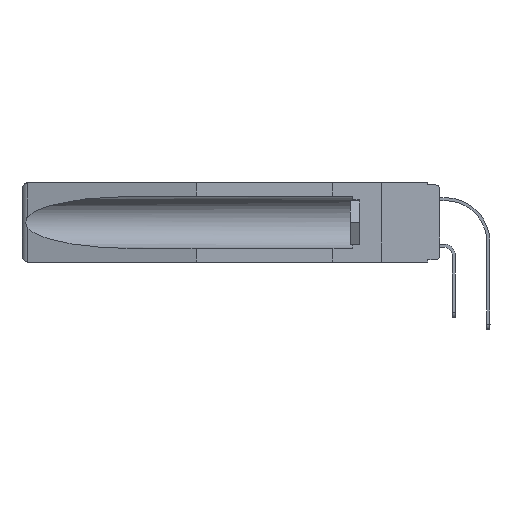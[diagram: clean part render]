
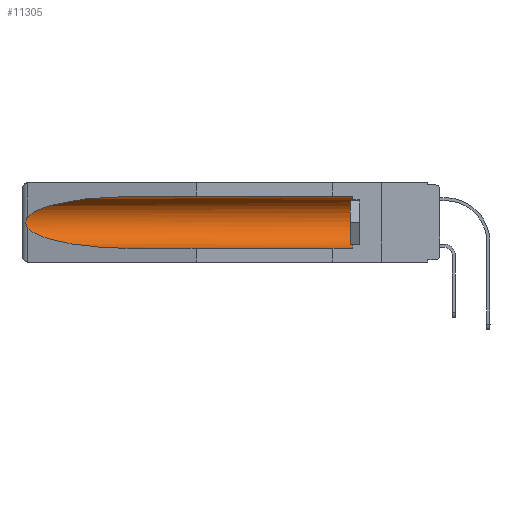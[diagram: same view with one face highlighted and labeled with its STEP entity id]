
A CAD part, left-side view. The second image highlights one B-rep face of the part: STEP entity #11305.
In plain terms, the highlighted cylindrical face has radius 2.857 mm (diameter 5.715 mm), a partial arc.
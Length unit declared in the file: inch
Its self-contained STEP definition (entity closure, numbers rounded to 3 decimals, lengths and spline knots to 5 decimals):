
#684 = CARTESIAN_POINT ( 'NONE',  ( 0.26597, 1.52961, -0.15275 ) ) ;
#916 = CARTESIAN_POINT ( 'NONE',  ( 0.26537, 1.52718, -0.19328 ) ) ;
#1855 = EDGE_CURVE ( 'NONE', #12677, #8878, #17461, .T. ) ;
#2428 = VECTOR ( 'NONE', #4899, 39.37008 ) ;
#2556 = VECTOR ( 'NONE', #22938, 39.37008 ) ;
#2964 = DIRECTION ( 'NONE',  ( 0., -1., 0. ) ) ;
#3357 = CARTESIAN_POINT ( 'NONE',  ( 0.26537, 1.52718, -0.14972 ) ) ;
#3511 = VERTEX_POINT ( 'NONE', #21932 ) ;
#4125 = CIRCLE ( 'NONE', #6401, 0.1125 ) ;
#4135 = EDGE_CURVE ( 'NONE', #6218, #3511, #13485, .T. ) ;
#4216 = CARTESIAN_POINT ( 'NONE',  ( 0.21114, 1.30732, -0.059 ) ) ;
#4338 = CARTESIAN_POINT ( 'NONE',  ( 0.25451, 1.48313, -0.09465 ) ) ;
#4899 = DIRECTION ( 'NONE',  ( 0., 1., 0. ) ) ;
#6130 = EDGE_CURVE ( 'NONE', #12677, #6218, #4125, .T. ) ;
#6218 = VERTEX_POINT ( 'NONE', #7567 ) ;
#6301 = CARTESIAN_POINT ( 'NONE',  ( 0.2673, 1.5327, -0.16383 ) ) ;
#6401 = AXIS2_PLACEMENT_3D ( 'NONE', #8334, #2964, #23059 ) ;
#6752 = CARTESIAN_POINT ( 'NONE',  ( 0.155, 0.126, -0.284 ) ) ;
#7068 = CARTESIAN_POINT ( 'NONE',  ( 0.21114, 1.30732, -0.284 ) ) ;
#7211 = ORIENTED_EDGE ( 'NONE', *, *, #4135, .T. ) ;
#7567 = CARTESIAN_POINT ( 'NONE',  ( 0.155, 0.126, -0.059 ) ) ;
#7980 = CARTESIAN_POINT ( 'NONE',  ( 0.26654, 1.53092, -0.15636 ) ) ;
#8334 = CARTESIAN_POINT ( 'NONE',  ( 0.155, 0.126, -0.1715 ) ) ;
#8448 = CARTESIAN_POINT ( 'NONE',  ( 0.155, -0.30754, -0.059 ) ) ;
#8683 = ORIENTED_EDGE ( 'NONE', *, *, #1855, .F. ) ;
#8878 = VERTEX_POINT ( 'NONE', #14005 ) ;
#8950 = VERTEX_POINT ( 'NONE', #3357 ) ;
#10060 = ORIENTED_EDGE ( 'NONE', *, *, #20190, .T. ) ;
#10434 = ORIENTED_EDGE ( 'NONE', *, *, #13040, .T. ) ;
#10481 = EDGE_LOOP ( 'NONE', ( #10434, #10060, #18855, #8683, #18354, #7211 ) ) ;
#11305 = ADVANCED_FACE ( 'NONE', ( #13354 ), #11776, .F. ) ;
#11628 = CARTESIAN_POINT ( 'NONE',  ( 0.26537, 1.52718, -0.14972 ) ) ;
#11776 = CYLINDRICAL_SURFACE ( 'NONE', #15337, 0.1125 ) ;
#11869 = CARTESIAN_POINT ( 'NONE',  ( 0.155, 1.07973, -0.059 ) ) ;
#12677 = VERTEX_POINT ( 'NONE', #6752 ) ;
#12902 = CARTESIAN_POINT ( 'NONE',  ( 0.26537, 1.52718, -0.19328 ) ) ;
#13040 = EDGE_CURVE ( 'NONE', #3511, #8950, #21766, .T. ) ;
#13354 = FACE_OUTER_BOUND ( 'NONE', #10481, .T. ) ;
#13461 = CARTESIAN_POINT ( 'NONE',  ( 0.155, -0.30754, -0.1715 ) ) ;
#13485 = LINE ( 'NONE', #8448, #2556 ) ;
#13492 = CARTESIAN_POINT ( 'NONE',  ( 0.26655, 1.53094, -0.18657 ) ) ;
#14005 = CARTESIAN_POINT ( 'NONE',  ( 0.155, 1.07973, -0.284 ) ) ;
#14249 = CARTESIAN_POINT ( 'NONE',  ( 0.155, 1.07973, -0.284 ) ) ;
#15279 = CARTESIAN_POINT ( 'NONE',  ( 0.2675, 1.53308, -0.16763 ) ) ;
#15337 = AXIS2_PLACEMENT_3D ( 'NONE', #13461, #15366, #20761 ) ;
#15366 = DIRECTION ( 'NONE',  ( 0., 1., 0. ) ) ;
#15400 = CARTESIAN_POINT ( 'NONE',  ( 0.26537, 1.52718, -0.14972 ) ) ;
#15928 = CARTESIAN_POINT ( 'NONE',  ( 0.26537, 1.52718, -0.19328 ) ) ;
#16098 =( BOUNDED_CURVE ( )  B_SPLINE_CURVE ( 3, ( #15928, #17968, #7068, #14249 ),
 .UNSPECIFIED., .F., .T. ) 
 B_SPLINE_CURVE_WITH_KNOTS ( ( 4, 4 ),
 ( 0.1948, 1.5708 ),
 .UNSPECIFIED. ) 
 CURVE ( )  GEOMETRIC_REPRESENTATION_ITEM ( )  RATIONAL_B_SPLINE_CURVE ( ( 1., 0.848, 0.848, 1. ) ) 
 REPRESENTATION_ITEM ( '' )  );
#17305 = CARTESIAN_POINT ( 'NONE',  ( 0.2675, 1.53308, -0.17534 ) ) ;
#17461 = LINE ( 'NONE', #19375, #2428 ) ;
#17968 = CARTESIAN_POINT ( 'NONE',  ( 0.25451, 1.48313, -0.24835 ) ) ;
#17988 = VERTEX_POINT ( 'NONE', #12902 ) ;
#18354 = ORIENTED_EDGE ( 'NONE', *, *, #6130, .T. ) ;
#18855 = ORIENTED_EDGE ( 'NONE', *, *, #19380, .T. ) ;
#19375 = CARTESIAN_POINT ( 'NONE',  ( 0.155, -0.30754, -0.284 ) ) ;
#19380 = EDGE_CURVE ( 'NONE', #17988, #8878, #16098, .T. ) ;
#20190 = EDGE_CURVE ( 'NONE', #8950, #17988, #22055, .T. ) ;
#20761 = DIRECTION ( 'NONE',  ( 0., 0., 1. ) ) ;
#21766 =( BOUNDED_CURVE ( )  B_SPLINE_CURVE ( 3, ( #11869, #4216, #4338, #11628 ),
 .UNSPECIFIED., .F., .T. ) 
 B_SPLINE_CURVE_WITH_KNOTS ( ( 4, 4 ),
 ( 4.71239, 6.08839 ),
 .UNSPECIFIED. ) 
 CURVE ( )  GEOMETRIC_REPRESENTATION_ITEM ( )  RATIONAL_B_SPLINE_CURVE ( ( 1., 0.848, 0.848, 1. ) ) 
 REPRESENTATION_ITEM ( '' )  );
#21932 = CARTESIAN_POINT ( 'NONE',  ( 0.155, 1.07973, -0.059 ) ) ;
#22055 = B_SPLINE_CURVE_WITH_KNOTS ( 'NONE', 3,
 ( #15400, #684, #7980, #6301, #15279, #17305, #22585, #13492, #22831, #916 ),
 .UNSPECIFIED., .F., .F.,
 ( 4, 2, 2, 2, 4 ),
 ( 0., 0.00029, 0.00058, 0.00087, 0.00117 ),
 .UNSPECIFIED. ) ;
#22585 = CARTESIAN_POINT ( 'NONE',  ( 0.2673, 1.53269, -0.17917 ) ) ;
#22831 = CARTESIAN_POINT ( 'NONE',  ( 0.26597, 1.5296, -0.19026 ) ) ;
#22938 = DIRECTION ( 'NONE',  ( 0., 1., 0. ) ) ;
#23059 = DIRECTION ( 'NONE',  ( 0., 0., 1. ) ) ;
